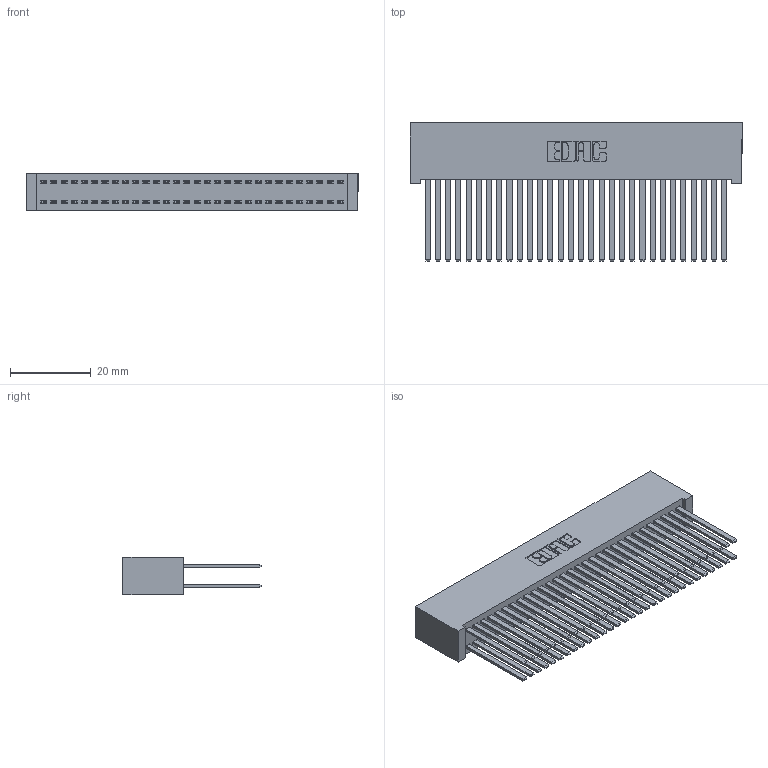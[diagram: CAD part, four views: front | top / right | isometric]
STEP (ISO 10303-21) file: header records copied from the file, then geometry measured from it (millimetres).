
FILE_DESCRIPTION (( 'STEP AP203' ), '1' );
FILE_NAME ('392-060-544-201.STEP', '2019-10-08T17:27:13', ( '' ), ( '' ), 'SwSTEP 2.0', 'SolidWorks 2016', '' );
FILE_SCHEMA (( 'CONFIG_CONTROL_DESIGN' ));
Length unit declared in the file: inch
Products named in the file (3): 342 Part_Lugless; 345-292-001_345-293-144; 392-060-544-201
Assembly tree (61 placements, depth 2):
  392-060-544-201
    342 Part_Lugless
    345-292-001_345-293-144  x60
Bounding box: 82.45 x 34.3 x 9.4 mm (x, y, z)
Volume: 8631.8 mm3; surface area: 16530.2 mm2
Topology: 61 solids, 61 shells, 2862 faces, 8495 edges, 5582 vertices
Faces by surface type: plane 1982, cylinder 880
Entity records: 20259 total; most frequent: CARTESIAN_POINT 3366, ORIENTED_EDGE 3302, DIRECTION 2887, EDGE_CURVE 1651, LINE 1535, VECTOR 1535, VERTEX_POINT 1098, AXIS2_PLACEMENT_3D 676
